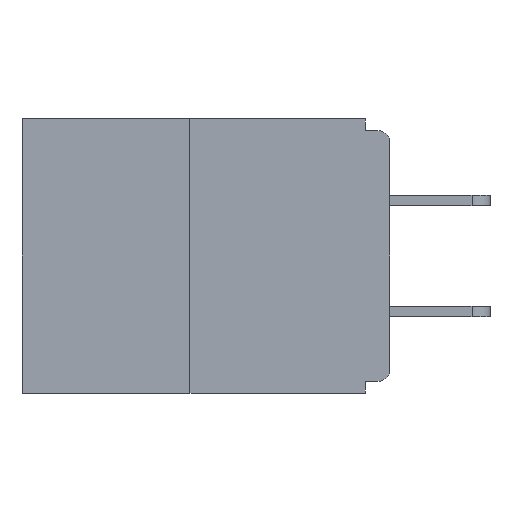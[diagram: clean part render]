
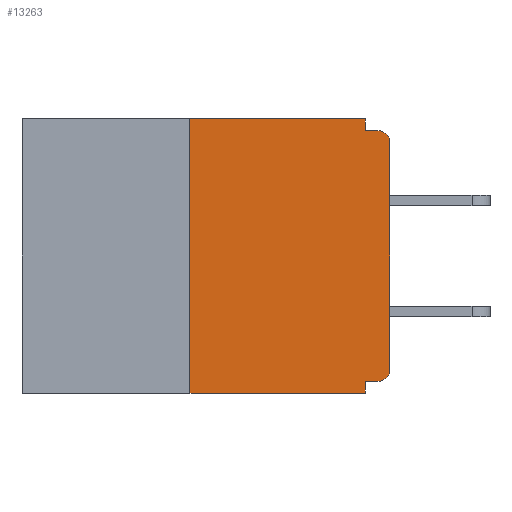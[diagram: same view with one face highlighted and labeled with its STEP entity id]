
A CAD part, left-side view. The second image highlights one B-rep face of the part: STEP entity #13263.
In plain terms, the highlighted planar face has unit normal (-1, 0, 0).
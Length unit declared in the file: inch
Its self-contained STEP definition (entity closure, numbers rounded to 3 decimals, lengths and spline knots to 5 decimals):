
#175 = EDGE_CURVE ( 'NONE', #240, #6335, #9798, .T. ) ;
#240 = VERTEX_POINT ( 'NONE', #14306 ) ;
#487 = VECTOR ( 'NONE', #574, 39.37008 ) ;
#574 = DIRECTION ( 'NONE',  ( 0., 0., 1. ) ) ;
#644 = ORIENTED_EDGE ( 'NONE', *, *, #1211, .T. ) ;
#1211 = EDGE_CURVE ( 'NONE', #4200, #10609, #26275, .T. ) ;
#1317 = VERTEX_POINT ( 'NONE', #19319 ) ;
#1485 = CARTESIAN_POINT ( 'NONE',  ( 0., 0.031, -0.343 ) ) ;
#1698 = DIRECTION ( 'NONE',  ( 0., -1., 0. ) ) ;
#2278 = CARTESIAN_POINT ( 'NONE',  ( 0., 0.25, -0.343 ) ) ;
#2556 = FACE_OUTER_BOUND ( 'NONE', #11477, .T. ) ;
#3497 = VECTOR ( 'NONE', #14853, 39.37008 ) ;
#3515 = DIRECTION ( 'NONE',  ( 0., 0., -1. ) ) ;
#3811 = VECTOR ( 'NONE', #5524, 39.37008 ) ;
#4200 = VERTEX_POINT ( 'NONE', #12493 ) ;
#5026 = EDGE_CURVE ( 'NONE', #19488, #19032, #19117, .T. ) ;
#5139 = LINE ( 'NONE', #6363, #3497 ) ;
#5311 = ORIENTED_EDGE ( 'NONE', *, *, #7599, .F. ) ;
#5420 = VECTOR ( 'NONE', #21330, 39.37008 ) ;
#5458 = ORIENTED_EDGE ( 'NONE', *, *, #19942, .T. ) ;
#5472 = DIRECTION ( 'NONE',  ( 1., 0., 0. ) ) ;
#5524 = DIRECTION ( 'NONE',  ( 0., 0., 1. ) ) ;
#5908 = AXIS2_PLACEMENT_3D ( 'NONE', #8584, #14832, #6428 ) ;
#6335 = VERTEX_POINT ( 'NONE', #26617 ) ;
#6363 = CARTESIAN_POINT ( 'NONE',  ( 0., 0.46, 0. ) ) ;
#6428 = DIRECTION ( 'NONE',  ( 0., 0., -1. ) ) ;
#6928 = CARTESIAN_POINT ( 'NONE',  ( 0., 0.031, 0. ) ) ;
#7599 = EDGE_CURVE ( 'NONE', #25961, #18942, #8773, .T. ) ;
#7941 = AXIS2_PLACEMENT_3D ( 'NONE', #14133, #5472, #3515 ) ;
#7956 = ORIENTED_EDGE ( 'NONE', *, *, #8063, .F. ) ;
#8037 = VECTOR ( 'NONE', #8625, 39.37008 ) ;
#8063 = EDGE_CURVE ( 'NONE', #1317, #19032, #20260, .T. ) ;
#8584 = CARTESIAN_POINT ( 'NONE',  ( 0., 0.015, -0.03 ) ) ;
#8625 = DIRECTION ( 'NONE',  ( 0., 1., 0. ) ) ;
#8773 = LINE ( 'NONE', #19315, #487 ) ;
#8930 = ORIENTED_EDGE ( 'NONE', *, *, #175, .F. ) ;
#9091 = ORIENTED_EDGE ( 'NONE', *, *, #9502, .F. ) ;
#9502 = EDGE_CURVE ( 'NONE', #4200, #240, #27161, .T. ) ;
#9798 = LINE ( 'NONE', #1485, #13750 ) ;
#10101 = LINE ( 'NONE', #11786, #3811 ) ;
#10379 = CARTESIAN_POINT ( 'NONE',  ( 0., 0.015, -0.313 ) ) ;
#10486 = DIRECTION ( 'NONE',  ( 0., 0., -1. ) ) ;
#10609 = VERTEX_POINT ( 'NONE', #15191 ) ;
#10618 = CARTESIAN_POINT ( 'NONE',  ( 0., 0.031, 0. ) ) ;
#10973 = CARTESIAN_POINT ( 'NONE',  ( 0., 0.015, -0.015 ) ) ;
#11477 = EDGE_LOOP ( 'NONE', ( #12707, #5311, #5458, #8930, #9091, #644, #26408, #16562, #7956, #27083 ) ) ;
#11786 = CARTESIAN_POINT ( 'NONE',  ( 0., 0., 0. ) ) ;
#12363 = AXIS2_PLACEMENT_3D ( 'NONE', #10379, #21265, #10486 ) ;
#12493 = CARTESIAN_POINT ( 'NONE',  ( 0., 0.015, -0.328 ) ) ;
#12707 = ORIENTED_EDGE ( 'NONE', *, *, #25190, .F. ) ;
#13263 = ADVANCED_FACE ( 'NONE', ( #2556 ), #26583, .F. ) ;
#13286 = CARTESIAN_POINT ( 'NONE',  ( 0., 0.25, 0. ) ) ;
#13393 = VERTEX_POINT ( 'NONE', #10618 ) ;
#13578 = VECTOR ( 'NONE', #17642, 39.37008 ) ;
#13750 = VECTOR ( 'NONE', #18465, 39.37008 ) ;
#14133 = CARTESIAN_POINT ( 'NONE',  ( 0., 0.46, 0. ) ) ;
#14245 = CARTESIAN_POINT ( 'NONE',  ( 0., 0.46, -0.343 ) ) ;
#14306 = CARTESIAN_POINT ( 'NONE',  ( 0., 0.031, -0.328 ) ) ;
#14832 = DIRECTION ( 'NONE',  ( -1., 0., 0. ) ) ;
#14853 = DIRECTION ( 'NONE',  ( 0., -1., 0. ) ) ;
#15191 = CARTESIAN_POINT ( 'NONE',  ( 0., 0., -0.313 ) ) ;
#16413 = LINE ( 'NONE', #14245, #20002 ) ;
#16562 = ORIENTED_EDGE ( 'NONE', *, *, #5026, .T. ) ;
#17642 = DIRECTION ( 'NONE',  ( 0., 0., -1. ) ) ;
#18465 = DIRECTION ( 'NONE',  ( 0., 0., -1. ) ) ;
#18942 = VERTEX_POINT ( 'NONE', #13286 ) ;
#19032 = VERTEX_POINT ( 'NONE', #10973 ) ;
#19117 = CIRCLE ( 'NONE', #5908, 0.015 ) ;
#19202 = CARTESIAN_POINT ( 'NONE',  ( 0., 0., -0.015 ) ) ;
#19315 = CARTESIAN_POINT ( 'NONE',  ( 0., 0.25, 0. ) ) ;
#19319 = CARTESIAN_POINT ( 'NONE',  ( 0., 0.031, -0.015 ) ) ;
#19488 = VERTEX_POINT ( 'NONE', #19962 ) ;
#19942 = EDGE_CURVE ( 'NONE', #25961, #6335, #16413, .T. ) ;
#19962 = CARTESIAN_POINT ( 'NONE',  ( 0., 0., -0.03 ) ) ;
#20002 = VECTOR ( 'NONE', #1698, 39.37008 ) ;
#20260 = LINE ( 'NONE', #19202, #5420 ) ;
#21036 = EDGE_CURVE ( 'NONE', #10609, #19488, #10101, .T. ) ;
#21265 = DIRECTION ( 'NONE',  ( -1., 0., 0. ) ) ;
#21330 = DIRECTION ( 'NONE',  ( 0., -1., 0. ) ) ;
#21523 = LINE ( 'NONE', #6928, #13578 ) ;
#21607 = CARTESIAN_POINT ( 'NONE',  ( 0., 0., -0.328 ) ) ;
#23306 = EDGE_CURVE ( 'NONE', #13393, #1317, #21523, .T. ) ;
#25190 = EDGE_CURVE ( 'NONE', #18942, #13393, #5139, .T. ) ;
#25961 = VERTEX_POINT ( 'NONE', #2278 ) ;
#26275 = CIRCLE ( 'NONE', #12363, 0.015 ) ;
#26408 = ORIENTED_EDGE ( 'NONE', *, *, #21036, .T. ) ;
#26583 = PLANE ( 'NONE',  #7941 ) ;
#26617 = CARTESIAN_POINT ( 'NONE',  ( 0., 0.031, -0.343 ) ) ;
#27083 = ORIENTED_EDGE ( 'NONE', *, *, #23306, .F. ) ;
#27161 = LINE ( 'NONE', #21607, #8037 ) ;
